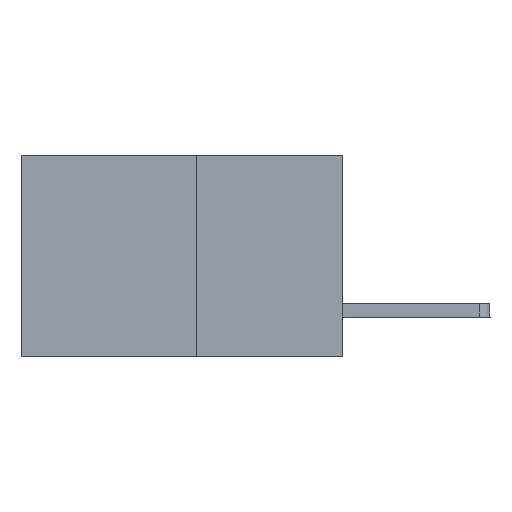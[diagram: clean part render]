
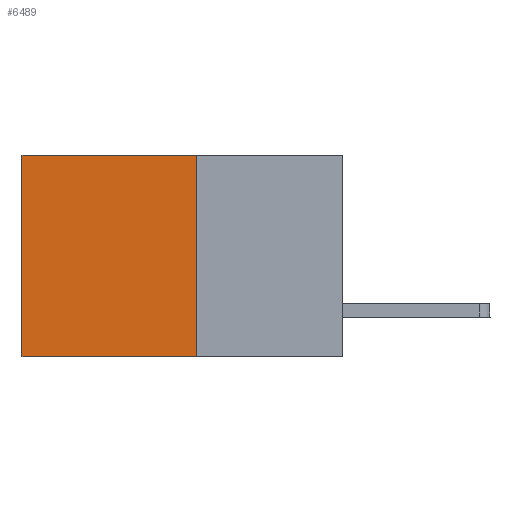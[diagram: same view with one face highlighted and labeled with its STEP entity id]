
A CAD part, left-side view. The second image highlights one B-rep face of the part: STEP entity #6489.
In plain terms, the highlighted planar face has unit normal (-1, 0, 0).
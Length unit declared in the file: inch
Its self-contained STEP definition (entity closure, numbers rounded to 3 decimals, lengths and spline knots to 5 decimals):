
#308 = ORIENTED_EDGE ( 'NONE', *, *, #6225, .F. ) ;
#572 = VERTEX_POINT ( 'NONE', #883 ) ;
#883 = CARTESIAN_POINT ( 'NONE',  ( 0.277, 0.27, -0.37 ) ) ;
#891 = VECTOR ( 'NONE', #906, 39.37008 ) ;
#906 = DIRECTION ( 'NONE',  ( 0., 0., -1. ) ) ;
#954 = EDGE_CURVE ( 'NONE', #10449, #2493, #1538, .T. ) ;
#1538 = LINE ( 'NONE', #12113, #8817 ) ;
#1893 = CARTESIAN_POINT ( 'NONE',  ( 0.277, 0.27, 0. ) ) ;
#2493 = VERTEX_POINT ( 'NONE', #4681 ) ;
#2562 = VECTOR ( 'NONE', #4116, 39.37008 ) ;
#2744 = PLANE ( 'NONE',  #9088 ) ;
#3674 = FACE_OUTER_BOUND ( 'NONE', #5559, .T. ) ;
#3925 = CARTESIAN_POINT ( 'NONE',  ( 0.277, 0.27, -0.37 ) ) ;
#4116 = DIRECTION ( 'NONE',  ( 0., 1., 0. ) ) ;
#4390 = EDGE_CURVE ( 'NONE', #2493, #10776, #10466, .T. ) ;
#4681 = CARTESIAN_POINT ( 'NONE',  ( 0.277, 0.59, 0. ) ) ;
#5222 = ORIENTED_EDGE ( 'NONE', *, *, #954, .T. ) ;
#5263 = DIRECTION ( 'NONE',  ( 0., 1., 0. ) ) ;
#5559 = EDGE_LOOP ( 'NONE', ( #9511, #308, #8951, #5222 ) ) ;
#6036 = CARTESIAN_POINT ( 'NONE',  ( 0.277, 0.59, -0.37 ) ) ;
#6225 = EDGE_CURVE ( 'NONE', #572, #10776, #8873, .T. ) ;
#6489 = ADVANCED_FACE ( 'NONE', ( #3674 ), #2744, .F. ) ;
#6894 = VECTOR ( 'NONE', #7517, 39.37008 ) ;
#7445 = DIRECTION ( 'NONE',  ( 0., 0., -1. ) ) ;
#7509 = CARTESIAN_POINT ( 'NONE',  ( 0.277, 0.27, -0.37 ) ) ;
#7517 = DIRECTION ( 'NONE',  ( 0., 0., -1. ) ) ;
#7563 = DIRECTION ( 'NONE',  ( 1., 0., 0. ) ) ;
#8817 = VECTOR ( 'NONE', #5263, 39.37008 ) ;
#8873 = LINE ( 'NONE', #3925, #2562 ) ;
#8951 = ORIENTED_EDGE ( 'NONE', *, *, #11305, .F. ) ;
#9088 = AXIS2_PLACEMENT_3D ( 'NONE', #7509, #7563, #7445 ) ;
#9511 = ORIENTED_EDGE ( 'NONE', *, *, #4390, .T. ) ;
#10366 = CARTESIAN_POINT ( 'NONE',  ( 0.277, 0.27, -0.37 ) ) ;
#10449 = VERTEX_POINT ( 'NONE', #1893 ) ;
#10466 = LINE ( 'NONE', #11337, #6894 ) ;
#10776 = VERTEX_POINT ( 'NONE', #6036 ) ;
#11223 = LINE ( 'NONE', #10366, #891 ) ;
#11305 = EDGE_CURVE ( 'NONE', #10449, #572, #11223, .T. ) ;
#11337 = CARTESIAN_POINT ( 'NONE',  ( 0.277, 0.59, -0.37 ) ) ;
#12113 = CARTESIAN_POINT ( 'NONE',  ( 0.277, 0.27, 0. ) ) ;
